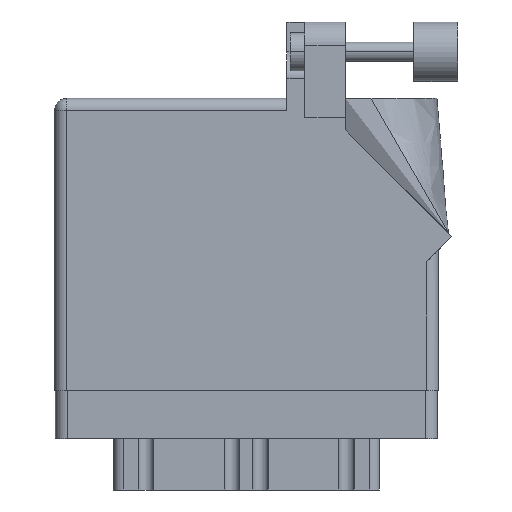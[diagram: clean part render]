
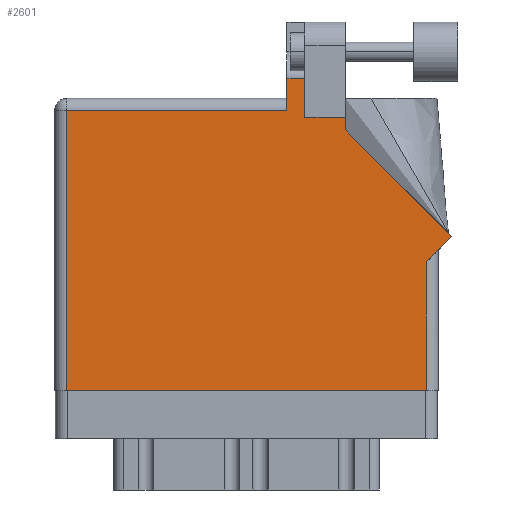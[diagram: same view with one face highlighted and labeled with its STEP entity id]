
A CAD part, front view. The second image highlights one B-rep face of the part: STEP entity #2601.
In plain terms, the highlighted face is planar.
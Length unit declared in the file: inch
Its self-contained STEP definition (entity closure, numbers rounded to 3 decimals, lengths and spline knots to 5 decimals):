
#79 = ORIENTED_EDGE ( 'NONE', *, *, #10465, .T. ) ;
#704 = VERTEX_POINT ( 'NONE', #8359 ) ;
#857 = CARTESIAN_POINT ( 'NONE',  ( 0., 1.53, 0. ) ) ;
#1664 = VECTOR ( 'NONE', #19654, 39.37008 ) ;
#2521 = ORIENTED_EDGE ( 'NONE', *, *, #11485, .T. ) ;
#2601 = ADVANCED_FACE ( 'NONE', ( #19902 ), #20089, .F. ) ;
#3608 = ORIENTED_EDGE ( 'NONE', *, *, #4930, .T. ) ;
#3793 = VERTEX_POINT ( 'NONE', #34707 ) ;
#4623 = CARTESIAN_POINT ( 'NONE',  ( 0.062, 1.468, 0. ) ) ;
#4644 = CARTESIAN_POINT ( 'NONE',  ( 0., 1.468, 0. ) ) ;
#4861 = VECTOR ( 'NONE', #32532, 39.37008 ) ;
#4896 = ORIENTED_EDGE ( 'NONE', *, *, #17452, .T. ) ;
#4930 = EDGE_CURVE ( 'NONE', #10346, #5434, #33638, .T. ) ;
#5144 = VECTOR ( 'NONE', #26561, 39.37008 ) ;
#5379 = VERTEX_POINT ( 'NONE', #22773 ) ;
#5434 = VERTEX_POINT ( 'NONE', #18471 ) ;
#5614 = AXIS2_PLACEMENT_3D ( 'NONE', #857, #17393, #31072 ) ;
#5942 = ORIENTED_EDGE ( 'NONE', *, *, #15334, .T. ) ;
#6380 = VECTOR ( 'NONE', #10708, 39.37008 ) ;
#6552 = LINE ( 'NONE', #33407, #13210 ) ;
#6625 = VERTEX_POINT ( 'NONE', #15112 ) ;
#6911 = DIRECTION ( 'NONE',  ( 0.707, 0.707, 0. ) ) ;
#7381 = EDGE_CURVE ( 'NONE', #30532, #6625, #28163, .T. ) ;
#7665 = CARTESIAN_POINT ( 'NONE',  ( 1.948, 0.737, 0. ) ) ;
#7951 = LINE ( 'NONE', #29135, #14445 ) ;
#7988 = CARTESIAN_POINT ( 'NONE',  ( 0.062, 0., 0. ) ) ;
#8359 = CARTESIAN_POINT ( 'NONE',  ( 1.311, 1.6315, 0. ) ) ;
#8485 = CARTESIAN_POINT ( 'NONE',  ( 2.08071, 0.80771, 0. ) ) ;
#8771 = DIRECTION ( 'NONE',  ( 1., 0., 0. ) ) ;
#9271 = CARTESIAN_POINT ( 'NONE',  ( 1.217, 1.53, 0. ) ) ;
#9348 = VERTEX_POINT ( 'NONE', #7988 ) ;
#10346 = VERTEX_POINT ( 'NONE', #28475 ) ;
#10465 = EDGE_CURVE ( 'NONE', #19138, #9348, #16014, .T. ) ;
#10708 = DIRECTION ( 'NONE',  ( 0., 1., 0. ) ) ;
#10896 = EDGE_CURVE ( 'NONE', #21785, #5379, #7951, .T. ) ;
#11269 = ORIENTED_EDGE ( 'NONE', *, *, #10896, .T. ) ;
#11279 = LINE ( 'NONE', #24634, #11912 ) ;
#11485 = EDGE_CURVE ( 'NONE', #9348, #3793, #11279, .T. ) ;
#11912 = VECTOR ( 'NONE', #8771, 39.37008 ) ;
#12680 = DIRECTION ( 'NONE',  ( 0., 1., 0. ) ) ;
#13210 = VECTOR ( 'NONE', #6911, 39.37008 ) ;
#14094 = CARTESIAN_POINT ( 'NONE',  ( 1.948, 0.675, 0. ) ) ;
#14445 = VECTOR ( 'NONE', #18649, 39.37008 ) ;
#14716 = VECTOR ( 'NONE', #26514, 39.37008 ) ;
#15112 = CARTESIAN_POINT ( 'NONE',  ( 1.311, 1.43, 0. ) ) ;
#15334 = EDGE_CURVE ( 'NONE', #5434, #19138, #15677, .T. ) ;
#15523 = LINE ( 'NONE', #7665, #34031 ) ;
#15677 = LINE ( 'NONE', #4644, #14716 ) ;
#16014 = LINE ( 'NONE', #21547, #4861 ) ;
#16673 = ORIENTED_EDGE ( 'NONE', *, *, #34107, .T. ) ;
#17393 = DIRECTION ( 'NONE',  ( 0., 0., -1. ) ) ;
#17452 = EDGE_CURVE ( 'NONE', #3793, #30021, #15523, .T. ) ;
#17606 = CARTESIAN_POINT ( 'NONE',  ( 1.524, 1.43, 0. ) ) ;
#17627 = DIRECTION ( 'NONE',  ( 0., 1., 0. ) ) ;
#18471 = CARTESIAN_POINT ( 'NONE',  ( 1.217, 1.468, 0. ) ) ;
#18649 = DIRECTION ( 'NONE',  ( -0.707, 0.707, 0. ) ) ;
#19011 = EDGE_CURVE ( 'NONE', #6625, #704, #27273, .T. ) ;
#19138 = VERTEX_POINT ( 'NONE', #4623 ) ;
#19654 = DIRECTION ( 'NONE',  ( -1., 0., 0. ) ) ;
#19902 = FACE_OUTER_BOUND ( 'NONE', #23750, .T. ) ;
#20089 = PLANE ( 'NONE',  #5614 ) ;
#20564 = EDGE_CURVE ( 'NONE', #5379, #30532, #32211, .T. ) ;
#20728 = ORIENTED_EDGE ( 'NONE', *, *, #31107, .T. ) ;
#21405 = CARTESIAN_POINT ( 'NONE',  ( 1.524, 1.36442, 0. ) ) ;
#21547 = CARTESIAN_POINT ( 'NONE',  ( 0.062, 0., 0. ) ) ;
#21785 = VERTEX_POINT ( 'NONE', #8485 ) ;
#22698 = ORIENTED_EDGE ( 'NONE', *, *, #19011, .T. ) ;
#22773 = CARTESIAN_POINT ( 'NONE',  ( 1.524, 1.36442, 0. ) ) ;
#23750 = EDGE_LOOP ( 'NONE', ( #22698, #20728, #3608, #5942, #79, #2521, #4896, #16673, #11269, #31985, #26337 ) ) ;
#24634 = CARTESIAN_POINT ( 'NONE',  ( 0., 0., 0. ) ) ;
#26337 = ORIENTED_EDGE ( 'NONE', *, *, #7381, .T. ) ;
#26514 = DIRECTION ( 'NONE',  ( -1., 0., 0. ) ) ;
#26561 = DIRECTION ( 'NONE',  ( -1., 0., 0. ) ) ;
#26983 = VECTOR ( 'NONE', #31138, 39.37008 ) ;
#27273 = LINE ( 'NONE', #31128, #34716 ) ;
#28163 = LINE ( 'NONE', #33325, #1664 ) ;
#28475 = CARTESIAN_POINT ( 'NONE',  ( 1.217, 1.6315, 0. ) ) ;
#29135 = CARTESIAN_POINT ( 'NONE',  ( 2.08071, 0.80771, 0. ) ) ;
#29229 = CARTESIAN_POINT ( 'NONE',  ( 1.64177, 1.6315, 0. ) ) ;
#30021 = VERTEX_POINT ( 'NONE', #14094 ) ;
#30532 = VERTEX_POINT ( 'NONE', #17606 ) ;
#31072 = DIRECTION ( 'NONE',  ( -1., 0., 0. ) ) ;
#31107 = EDGE_CURVE ( 'NONE', #704, #10346, #32586, .T. ) ;
#31128 = CARTESIAN_POINT ( 'NONE',  ( 1.311, 1.43, 0. ) ) ;
#31138 = DIRECTION ( 'NONE',  ( 0., -1., 0. ) ) ;
#31985 = ORIENTED_EDGE ( 'NONE', *, *, #20564, .T. ) ;
#32211 = LINE ( 'NONE', #21405, #6380 ) ;
#32532 = DIRECTION ( 'NONE',  ( 0., -1., 0. ) ) ;
#32586 = LINE ( 'NONE', #29229, #5144 ) ;
#33325 = CARTESIAN_POINT ( 'NONE',  ( 1.524, 1.43, 0. ) ) ;
#33407 = CARTESIAN_POINT ( 'NONE',  ( 2.01, 0.737, 0. ) ) ;
#33638 = LINE ( 'NONE', #9271, #26983 ) ;
#34031 = VECTOR ( 'NONE', #12680, 39.37008 ) ;
#34107 = EDGE_CURVE ( 'NONE', #30021, #21785, #6552, .T. ) ;
#34707 = CARTESIAN_POINT ( 'NONE',  ( 1.948, 0., 0. ) ) ;
#34716 = VECTOR ( 'NONE', #17627, 39.37008 ) ;
